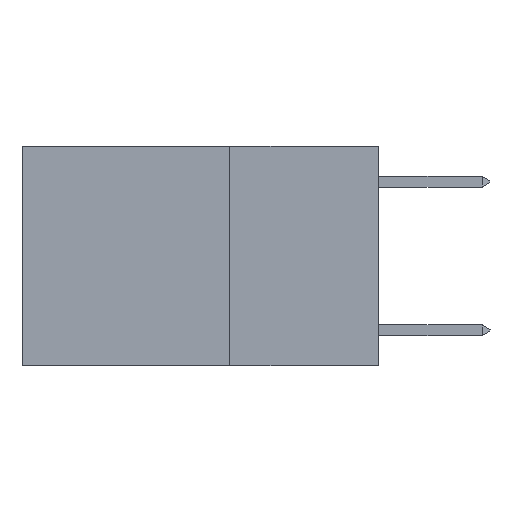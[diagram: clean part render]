
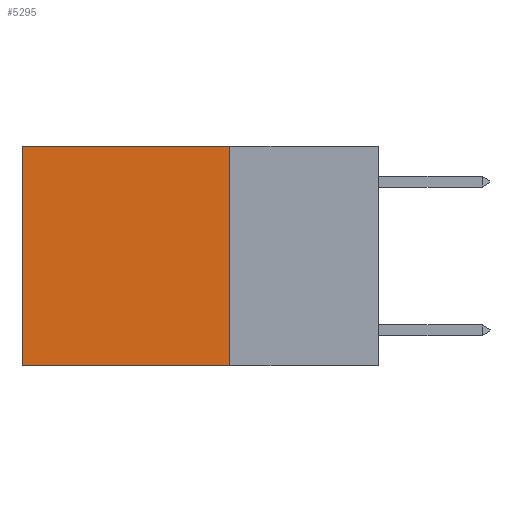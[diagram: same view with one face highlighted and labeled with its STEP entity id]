
A CAD part, left-side view. The second image highlights one B-rep face of the part: STEP entity #5295.
In plain terms, the highlighted planar face has unit normal (-1, 0, 0).
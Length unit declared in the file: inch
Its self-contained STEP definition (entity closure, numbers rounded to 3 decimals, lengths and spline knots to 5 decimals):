
#415 = CARTESIAN_POINT ( 'NONE',  ( 0.2625, 0.25, -0.37 ) ) ;
#462 = DIRECTION ( 'NONE',  ( 1., 0., 0. ) ) ;
#1344 = EDGE_CURVE ( 'NONE', #10710, #2925, #2438, .T. ) ;
#1700 = CARTESIAN_POINT ( 'NONE',  ( 0.2625, 0.25, 0. ) ) ;
#2062 = VECTOR ( 'NONE', #16025, 39.37008 ) ;
#2276 = CARTESIAN_POINT ( 'NONE',  ( 0.2625, 0.6, 0. ) ) ;
#2438 = LINE ( 'NONE', #2276, #10725 ) ;
#2455 = LINE ( 'NONE', #4415, #2062 ) ;
#2833 = DIRECTION ( 'NONE',  ( 0., 0., -1. ) ) ;
#2925 = VERTEX_POINT ( 'NONE', #12274 ) ;
#4292 = VECTOR ( 'NONE', #10677, 39.37008 ) ;
#4415 = CARTESIAN_POINT ( 'NONE',  ( 0.2625, 0.25, 0. ) ) ;
#5295 = ADVANCED_FACE ( 'NONE', ( #8609 ), #14573, .F. ) ;
#6430 = VERTEX_POINT ( 'NONE', #7635 ) ;
#6458 = ORIENTED_EDGE ( 'NONE', *, *, #1344, .T. ) ;
#6855 = CARTESIAN_POINT ( 'NONE',  ( 0.2625, 0.25, 0. ) ) ;
#7289 = AXIS2_PLACEMENT_3D ( 'NONE', #6855, #462, #2833 ) ;
#7635 = CARTESIAN_POINT ( 'NONE',  ( 0.2625, 0.25, 0. ) ) ;
#7771 = EDGE_CURVE ( 'NONE', #6430, #10415, #2455, .T. ) ;
#8148 = LINE ( 'NONE', #1700, #4292 ) ;
#8609 = FACE_OUTER_BOUND ( 'NONE', #10390, .T. ) ;
#8783 = DIRECTION ( 'NONE',  ( 0., 0., -1. ) ) ;
#10390 = EDGE_LOOP ( 'NONE', ( #6458, #16452, #10652, #13497 ) ) ;
#10415 = VERTEX_POINT ( 'NONE', #14474 ) ;
#10652 = ORIENTED_EDGE ( 'NONE', *, *, #7771, .F. ) ;
#10677 = DIRECTION ( 'NONE',  ( 0., 1., 0. ) ) ;
#10710 = VERTEX_POINT ( 'NONE', #14784 ) ;
#10725 = VECTOR ( 'NONE', #8783, 39.37008 ) ;
#10997 = EDGE_CURVE ( 'NONE', #10415, #2925, #13759, .T. ) ;
#12274 = CARTESIAN_POINT ( 'NONE',  ( 0.2625, 0.6, -0.37 ) ) ;
#12937 = VECTOR ( 'NONE', #13179, 39.37008 ) ;
#13179 = DIRECTION ( 'NONE',  ( 0., 1., 0. ) ) ;
#13497 = ORIENTED_EDGE ( 'NONE', *, *, #15396, .T. ) ;
#13759 = LINE ( 'NONE', #415, #12937 ) ;
#14474 = CARTESIAN_POINT ( 'NONE',  ( 0.2625, 0.25, -0.37 ) ) ;
#14573 = PLANE ( 'NONE',  #7289 ) ;
#14784 = CARTESIAN_POINT ( 'NONE',  ( 0.2625, 0.6, 0. ) ) ;
#15396 = EDGE_CURVE ( 'NONE', #6430, #10710, #8148, .T. ) ;
#16025 = DIRECTION ( 'NONE',  ( 0., 0., -1. ) ) ;
#16452 = ORIENTED_EDGE ( 'NONE', *, *, #10997, .F. ) ;
